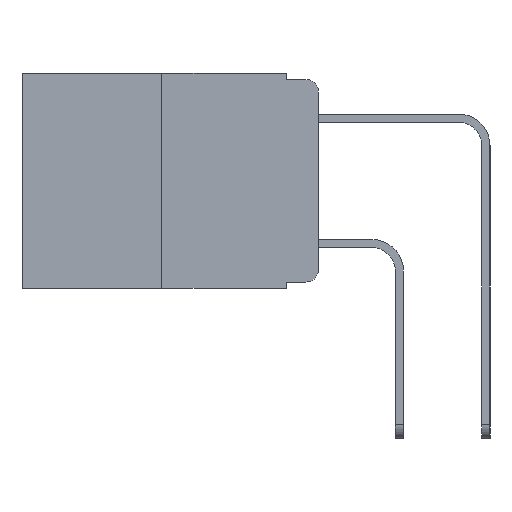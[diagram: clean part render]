
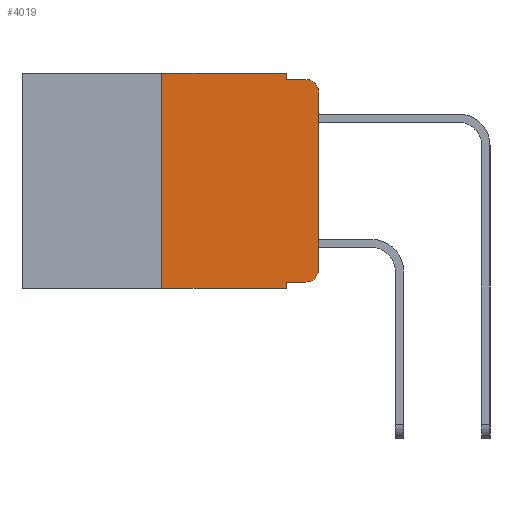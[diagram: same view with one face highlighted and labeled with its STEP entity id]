
A CAD part, left-side view. The second image highlights one B-rep face of the part: STEP entity #4019.
In plain terms, the highlighted planar face has unit normal (-1, 0, 0).
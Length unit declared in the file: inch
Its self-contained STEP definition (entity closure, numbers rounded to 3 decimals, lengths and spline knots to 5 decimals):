
#120 = ORIENTED_EDGE ( 'NONE', *, *, #15503, .T. ) ;
#329 = VECTOR ( 'NONE', #398, 39.37008 ) ;
#398 = DIRECTION ( 'NONE',  ( 0., 0., -1. ) ) ;
#1077 = CARTESIAN_POINT ( 'NONE',  ( 0., 0.25, 0. ) ) ;
#1436 = ORIENTED_EDGE ( 'NONE', *, *, #4411, .T. ) ;
#1440 = VERTEX_POINT ( 'NONE', #18118 ) ;
#1484 = CARTESIAN_POINT ( 'NONE',  ( 0., 0., -0.03 ) ) ;
#1630 = ORIENTED_EDGE ( 'NONE', *, *, #10026, .T. ) ;
#2389 = LINE ( 'NONE', #16178, #6614 ) ;
#2437 = EDGE_CURVE ( 'NONE', #1440, #22344, #5404, .T. ) ;
#2555 = VERTEX_POINT ( 'NONE', #17614 ) ;
#2657 = DIRECTION ( 'NONE',  ( -1., 0., 0. ) ) ;
#3062 = VERTEX_POINT ( 'NONE', #22222 ) ;
#3274 = VERTEX_POINT ( 'NONE', #14134 ) ;
#3858 = EDGE_CURVE ( 'NONE', #4889, #3062, #6448, .T. ) ;
#4019 = ADVANCED_FACE ( 'NONE', ( #20212 ), #22852, .F. ) ;
#4191 = VERTEX_POINT ( 'NONE', #20325 ) ;
#4234 = ORIENTED_EDGE ( 'NONE', *, *, #18294, .F. ) ;
#4411 = EDGE_CURVE ( 'NONE', #12903, #4191, #8408, .T. ) ;
#4556 = ORIENTED_EDGE ( 'NONE', *, *, #16095, .F. ) ;
#4784 = VECTOR ( 'NONE', #19149, 39.37008 ) ;
#4889 = VERTEX_POINT ( 'NONE', #10144 ) ;
#5404 = LINE ( 'NONE', #19052, #14898 ) ;
#5420 = VECTOR ( 'NONE', #9730, 39.37008 ) ;
#6448 = LINE ( 'NONE', #10350, #4784 ) ;
#6514 = DIRECTION ( 'NONE',  ( 0., -1., 0. ) ) ;
#6553 = DIRECTION ( 'NONE',  ( 0., 0., 1. ) ) ;
#6614 = VECTOR ( 'NONE', #14395, 39.37008 ) ;
#6670 = ORIENTED_EDGE ( 'NONE', *, *, #7319, .F. ) ;
#7014 = DIRECTION ( 'NONE',  ( -1., 0., 0. ) ) ;
#7319 = EDGE_CURVE ( 'NONE', #1440, #2555, #12698, .T. ) ;
#7581 = ORIENTED_EDGE ( 'NONE', *, *, #8248, .F. ) ;
#7752 = LINE ( 'NONE', #17087, #21159 ) ;
#8248 = EDGE_CURVE ( 'NONE', #2555, #21954, #2389, .T. ) ;
#8408 = CIRCLE ( 'NONE', #9961, 0.02 ) ;
#8537 = DIRECTION ( 'NONE',  ( 0., -1., 0. ) ) ;
#9410 = ORIENTED_EDGE ( 'NONE', *, *, #14307, .F. ) ;
#9730 = DIRECTION ( 'NONE',  ( 0., 0., -1. ) ) ;
#9961 = AXIS2_PLACEMENT_3D ( 'NONE', #17615, #7014, #19350 ) ;
#10026 = EDGE_CURVE ( 'NONE', #14174, #12903, #16553, .T. ) ;
#10144 = CARTESIAN_POINT ( 'NONE',  ( 0., 0.051, -0.333 ) ) ;
#10350 = CARTESIAN_POINT ( 'NONE',  ( 0., 0.051, -0.333 ) ) ;
#10797 = CARTESIAN_POINT ( 'NONE',  ( 0., 0.473, 0. ) ) ;
#10959 = CARTESIAN_POINT ( 'NONE',  ( 0., 0.051, 0. ) ) ;
#12561 = DIRECTION ( 'NONE',  ( 0., 0., -1. ) ) ;
#12633 = ORIENTED_EDGE ( 'NONE', *, *, #3858, .T. ) ;
#12698 = LINE ( 'NONE', #1077, #16837 ) ;
#12746 = AXIS2_PLACEMENT_3D ( 'NONE', #13367, #2657, #15173 ) ;
#12903 = VERTEX_POINT ( 'NONE', #1484 ) ;
#13367 = CARTESIAN_POINT ( 'NONE',  ( 0., 0.02, -0.313 ) ) ;
#14037 = ORIENTED_EDGE ( 'NONE', *, *, #2437, .T. ) ;
#14134 = CARTESIAN_POINT ( 'NONE',  ( 0., 0.051, -0.01 ) ) ;
#14174 = VERTEX_POINT ( 'NONE', #18094 ) ;
#14307 = EDGE_CURVE ( 'NONE', #21954, #3274, #19498, .T. ) ;
#14379 = AXIS2_PLACEMENT_3D ( 'NONE', #10797, #22922, #12561 ) ;
#14395 = DIRECTION ( 'NONE',  ( 0., -1., 0. ) ) ;
#14898 = VECTOR ( 'NONE', #8537, 39.37008 ) ;
#15173 = DIRECTION ( 'NONE',  ( 0., 0., -1. ) ) ;
#15503 = EDGE_CURVE ( 'NONE', #3062, #14174, #17559, .T. ) ;
#16095 = EDGE_CURVE ( 'NONE', #4889, #22344, #19414, .T. ) ;
#16178 = CARTESIAN_POINT ( 'NONE',  ( 0., 0.473, 0. ) ) ;
#16553 = LINE ( 'NONE', #21189, #20557 ) ;
#16837 = VECTOR ( 'NONE', #6553, 39.37008 ) ;
#17087 = CARTESIAN_POINT ( 'NONE',  ( 0., 0.051, -0.01 ) ) ;
#17559 = CIRCLE ( 'NONE', #12746, 0.02 ) ;
#17614 = CARTESIAN_POINT ( 'NONE',  ( 0., 0.25, 0. ) ) ;
#17615 = CARTESIAN_POINT ( 'NONE',  ( 0., 0.02, -0.03 ) ) ;
#17832 = DIRECTION ( 'NONE',  ( 0., 0., 1. ) ) ;
#18094 = CARTESIAN_POINT ( 'NONE',  ( 0., 0., -0.313 ) ) ;
#18118 = CARTESIAN_POINT ( 'NONE',  ( 0., 0.25, -0.343 ) ) ;
#18294 = EDGE_CURVE ( 'NONE', #3274, #4191, #7752, .T. ) ;
#19052 = CARTESIAN_POINT ( 'NONE',  ( 0., 0.473, -0.343 ) ) ;
#19149 = DIRECTION ( 'NONE',  ( 0., -1., 0. ) ) ;
#19350 = DIRECTION ( 'NONE',  ( 0., 0., -1. ) ) ;
#19414 = LINE ( 'NONE', #21757, #329 ) ;
#19498 = LINE ( 'NONE', #21901, #5420 ) ;
#20212 = FACE_OUTER_BOUND ( 'NONE', #21453, .T. ) ;
#20325 = CARTESIAN_POINT ( 'NONE',  ( 0., 0.02, -0.01 ) ) ;
#20557 = VECTOR ( 'NONE', #17832, 39.37008 ) ;
#20764 = CARTESIAN_POINT ( 'NONE',  ( 0., 0.051, -0.343 ) ) ;
#21159 = VECTOR ( 'NONE', #6514, 39.37008 ) ;
#21189 = CARTESIAN_POINT ( 'NONE',  ( 0., 0., 0. ) ) ;
#21453 = EDGE_LOOP ( 'NONE', ( #1630, #1436, #4234, #9410, #7581, #6670, #14037, #4556, #12633, #120 ) ) ;
#21757 = CARTESIAN_POINT ( 'NONE',  ( 0., 0.051, 0. ) ) ;
#21901 = CARTESIAN_POINT ( 'NONE',  ( 0., 0.051, 0. ) ) ;
#21954 = VERTEX_POINT ( 'NONE', #10959 ) ;
#22222 = CARTESIAN_POINT ( 'NONE',  ( 0., 0.02, -0.333 ) ) ;
#22344 = VERTEX_POINT ( 'NONE', #20764 ) ;
#22852 = PLANE ( 'NONE',  #14379 ) ;
#22922 = DIRECTION ( 'NONE',  ( 1., 0., 0. ) ) ;
